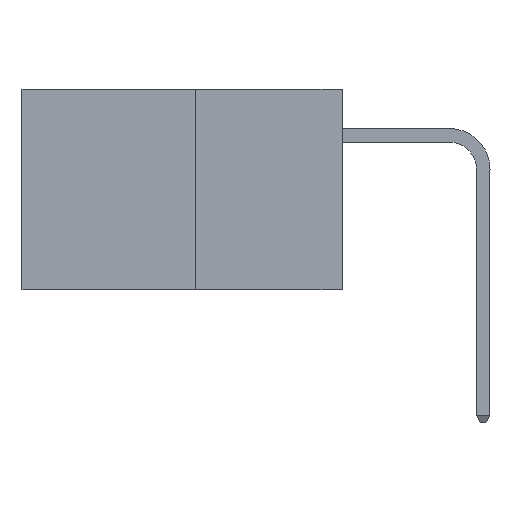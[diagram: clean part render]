
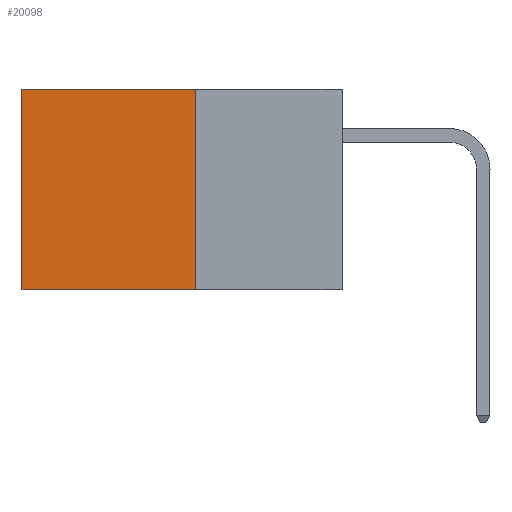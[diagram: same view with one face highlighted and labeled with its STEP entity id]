
A CAD part, left-side view. The second image highlights one B-rep face of the part: STEP entity #20098.
In plain terms, the highlighted planar face has unit normal (-1, 0, 0).
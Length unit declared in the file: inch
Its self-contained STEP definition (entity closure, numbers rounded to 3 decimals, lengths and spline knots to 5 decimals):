
#1451 = VERTEX_POINT ( 'NONE', #4813 ) ;
#1859 = LINE ( 'NONE', #11599, #15275 ) ;
#2069 = ORIENTED_EDGE ( 'NONE', *, *, #21821, .T. ) ;
#2364 = CARTESIAN_POINT ( 'NONE',  ( 0.277, 0.27, 0. ) ) ;
#2621 = LINE ( 'NONE', #18648, #11994 ) ;
#4813 = CARTESIAN_POINT ( 'NONE',  ( 0.277, 0.59, 0. ) ) ;
#5594 = LINE ( 'NONE', #8276, #14228 ) ;
#6341 = ORIENTED_EDGE ( 'NONE', *, *, #7295, .F. ) ;
#7295 = EDGE_CURVE ( 'NONE', #16867, #16061, #2621, .T. ) ;
#7304 = DIRECTION ( 'NONE',  ( 0., 0., -1. ) ) ;
#8276 = CARTESIAN_POINT ( 'NONE',  ( 0.277, 0.27, 0. ) ) ;
#8379 = DIRECTION ( 'NONE',  ( 0., 1., 0. ) ) ;
#10049 = DIRECTION ( 'NONE',  ( 0., 0., -1. ) ) ;
#10471 = VERTEX_POINT ( 'NONE', #2364 ) ;
#11594 = FACE_OUTER_BOUND ( 'NONE', #12899, .T. ) ;
#11599 = CARTESIAN_POINT ( 'NONE',  ( 0.277, 0.59, -0.37 ) ) ;
#11994 = VECTOR ( 'NONE', #8379, 39.37008 ) ;
#12899 = EDGE_LOOP ( 'NONE', ( #2069, #6341, #21675, #19615 ) ) ;
#13135 = EDGE_CURVE ( 'NONE', #10471, #16867, #17718, .T. ) ;
#13359 = CARTESIAN_POINT ( 'NONE',  ( 0.277, 0.59, -0.37 ) ) ;
#13469 = EDGE_CURVE ( 'NONE', #10471, #1451, #5594, .T. ) ;
#14228 = VECTOR ( 'NONE', #21950, 39.37008 ) ;
#15095 = CARTESIAN_POINT ( 'NONE',  ( 0.277, 0.27, -0.37 ) ) ;
#15275 = VECTOR ( 'NONE', #18473, 39.37008 ) ;
#16061 = VERTEX_POINT ( 'NONE', #13359 ) ;
#16867 = VERTEX_POINT ( 'NONE', #17203 ) ;
#17176 = VECTOR ( 'NONE', #7304, 39.37008 ) ;
#17203 = CARTESIAN_POINT ( 'NONE',  ( 0.277, 0.27, -0.37 ) ) ;
#17718 = LINE ( 'NONE', #21002, #17176 ) ;
#18473 = DIRECTION ( 'NONE',  ( 0., 0., -1. ) ) ;
#18648 = CARTESIAN_POINT ( 'NONE',  ( 0.277, 0.27, -0.37 ) ) ;
#19615 = ORIENTED_EDGE ( 'NONE', *, *, #13469, .T. ) ;
#19950 = AXIS2_PLACEMENT_3D ( 'NONE', #15095, #20257, #10049 ) ;
#20098 = ADVANCED_FACE ( 'NONE', ( #11594 ), #21880, .F. ) ;
#20257 = DIRECTION ( 'NONE',  ( 1., 0., 0. ) ) ;
#21002 = CARTESIAN_POINT ( 'NONE',  ( 0.277, 0.27, -0.37 ) ) ;
#21675 = ORIENTED_EDGE ( 'NONE', *, *, #13135, .F. ) ;
#21821 = EDGE_CURVE ( 'NONE', #1451, #16061, #1859, .T. ) ;
#21880 = PLANE ( 'NONE',  #19950 ) ;
#21950 = DIRECTION ( 'NONE',  ( 0., 1., 0. ) ) ;
